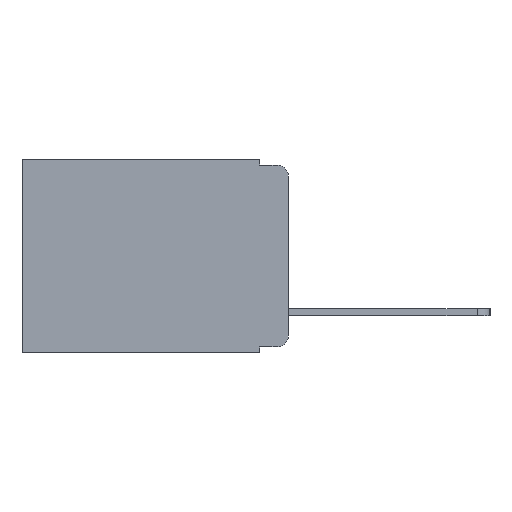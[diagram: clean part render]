
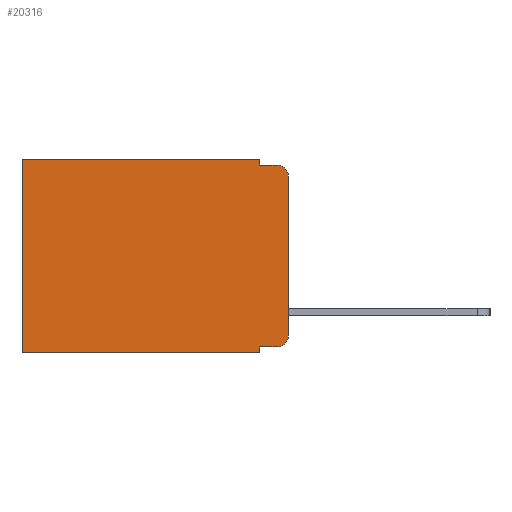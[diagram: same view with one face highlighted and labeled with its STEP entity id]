
A CAD part, left-side view. The second image highlights one B-rep face of the part: STEP entity #20316.
In plain terms, the highlighted planar face has unit normal (-1, 0, 0).
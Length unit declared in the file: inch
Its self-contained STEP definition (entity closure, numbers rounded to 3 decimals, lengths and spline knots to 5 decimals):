
#592 = ORIENTED_EDGE ( 'NONE', *, *, #4525, .F. ) ;
#769 = EDGE_CURVE ( 'NONE', #2695, #11790, #1768, .T. ) ;
#1333 = EDGE_CURVE ( 'NONE', #11790, #14523, #2235, .T. ) ;
#1568 = VECTOR ( 'NONE', #18440, 39.37008 ) ;
#1768 = LINE ( 'NONE', #15369, #18785 ) ;
#1835 = VECTOR ( 'NONE', #19156, 39.37008 ) ;
#2235 = LINE ( 'NONE', #2574, #6680 ) ;
#2326 = VERTEX_POINT ( 'NONE', #19909 ) ;
#2427 = VERTEX_POINT ( 'NONE', #18891 ) ;
#2574 = CARTESIAN_POINT ( 'NONE',  ( 0.298, 0., -0.343 ) ) ;
#2676 = DIRECTION ( 'NONE',  ( -1., 0., 0. ) ) ;
#2695 = VERTEX_POINT ( 'NONE', #8206 ) ;
#2753 = AXIS2_PLACEMENT_3D ( 'NONE', #18118, #8752, #19669 ) ;
#2941 = ORIENTED_EDGE ( 'NONE', *, *, #13127, .T. ) ;
#2972 = CIRCLE ( 'NONE', #10777, 0.02 ) ;
#3324 = DIRECTION ( 'NONE',  ( 1., 0., 0. ) ) ;
#3425 = ORIENTED_EDGE ( 'NONE', *, *, #16309, .T. ) ;
#3449 = CARTESIAN_POINT ( 'NONE',  ( 0.298, 0., 0. ) ) ;
#4099 = VECTOR ( 'NONE', #15192, 39.37008 ) ;
#4525 = EDGE_CURVE ( 'NONE', #5292, #13563, #7042, .T. ) ;
#4908 = DIRECTION ( 'NONE',  ( 0., 1., 0. ) ) ;
#5045 = ORIENTED_EDGE ( 'NONE', *, *, #5663, .F. ) ;
#5182 = PLANE ( 'NONE',  #19134 ) ;
#5292 = VERTEX_POINT ( 'NONE', #13034 ) ;
#5663 = EDGE_CURVE ( 'NONE', #17700, #12275, #8539, .T. ) ;
#6520 = VERTEX_POINT ( 'NONE', #13175 ) ;
#6633 = CARTESIAN_POINT ( 'NONE',  ( 0.298, 0.051, 0. ) ) ;
#6680 = VECTOR ( 'NONE', #4908, 39.37008 ) ;
#6870 = DIRECTION ( 'NONE',  ( 0., 0., -1. ) ) ;
#6920 = CARTESIAN_POINT ( 'NONE',  ( 0.298, 0., 0. ) ) ;
#7042 = LINE ( 'NONE', #10525, #1568 ) ;
#7335 = CARTESIAN_POINT ( 'NONE',  ( 0.298, 0.051, -0.333 ) ) ;
#7378 = CARTESIAN_POINT ( 'NONE',  ( 0.298, 0.051, -0.01 ) ) ;
#7644 = LINE ( 'NONE', #13726, #8873 ) ;
#7738 = LINE ( 'NONE', #7335, #19713 ) ;
#7903 = EDGE_CURVE ( 'NONE', #5292, #12275, #2972, .T. ) ;
#8206 = CARTESIAN_POINT ( 'NONE',  ( 0.298, 0.051, -0.333 ) ) ;
#8539 = LINE ( 'NONE', #7378, #4099 ) ;
#8565 = EDGE_CURVE ( 'NONE', #2326, #13563, #13370, .T. ) ;
#8752 = DIRECTION ( 'NONE',  ( -1., 0., 0. ) ) ;
#8873 = VECTOR ( 'NONE', #18473, 39.37008 ) ;
#9312 = FACE_OUTER_BOUND ( 'NONE', #13287, .T. ) ;
#9559 = CARTESIAN_POINT ( 'NONE',  ( 0.298, 0.473, -0.343 ) ) ;
#10337 = ORIENTED_EDGE ( 'NONE', *, *, #1333, .F. ) ;
#10525 = CARTESIAN_POINT ( 'NONE',  ( 0.298, 0., 0. ) ) ;
#10777 = AXIS2_PLACEMENT_3D ( 'NONE', #12347, #2676, #13936 ) ;
#10828 = ORIENTED_EDGE ( 'NONE', *, *, #8565, .T. ) ;
#10952 = CARTESIAN_POINT ( 'NONE',  ( 0.298, 0.051, -0.343 ) ) ;
#11535 = ORIENTED_EDGE ( 'NONE', *, *, #769, .F. ) ;
#11790 = VERTEX_POINT ( 'NONE', #10952 ) ;
#12275 = VERTEX_POINT ( 'NONE', #13337 ) ;
#12347 = CARTESIAN_POINT ( 'NONE',  ( 0.298, 0.02, -0.03 ) ) ;
#13034 = CARTESIAN_POINT ( 'NONE',  ( 0.298, 0., -0.03 ) ) ;
#13127 = EDGE_CURVE ( 'NONE', #2427, #14523, #7644, .T. ) ;
#13175 = CARTESIAN_POINT ( 'NONE',  ( 0.298, 0.051, 0. ) ) ;
#13287 = EDGE_LOOP ( 'NONE', ( #592, #15228, #5045, #15722, #13524, #2941, #10337, #11535, #3425, #10828 ) ) ;
#13337 = CARTESIAN_POINT ( 'NONE',  ( 0.298, 0.02, -0.01 ) ) ;
#13370 = CIRCLE ( 'NONE', #2753, 0.02 ) ;
#13524 = ORIENTED_EDGE ( 'NONE', *, *, #19018, .T. ) ;
#13563 = VERTEX_POINT ( 'NONE', #14945 ) ;
#13726 = CARTESIAN_POINT ( 'NONE',  ( 0.298, 0.473, 0. ) ) ;
#13936 = DIRECTION ( 'NONE',  ( 0., 0., -1. ) ) ;
#14523 = VERTEX_POINT ( 'NONE', #9559 ) ;
#14680 = LINE ( 'NONE', #6633, #1835 ) ;
#14754 = VECTOR ( 'NONE', #16418, 39.37008 ) ;
#14945 = CARTESIAN_POINT ( 'NONE',  ( 0.298, 0., -0.313 ) ) ;
#15192 = DIRECTION ( 'NONE',  ( 0., -1., 0. ) ) ;
#15228 = ORIENTED_EDGE ( 'NONE', *, *, #7903, .T. ) ;
#15241 = EDGE_CURVE ( 'NONE', #6520, #17700, #14680, .T. ) ;
#15369 = CARTESIAN_POINT ( 'NONE',  ( 0.298, 0.051, 0. ) ) ;
#15722 = ORIENTED_EDGE ( 'NONE', *, *, #15241, .F. ) ;
#16309 = EDGE_CURVE ( 'NONE', #2695, #2326, #7738, .T. ) ;
#16418 = DIRECTION ( 'NONE',  ( 0., 1., 0. ) ) ;
#16641 = DIRECTION ( 'NONE',  ( 0., 0., -1. ) ) ;
#17152 = CARTESIAN_POINT ( 'NONE',  ( 0.298, 0.051, -0.01 ) ) ;
#17700 = VERTEX_POINT ( 'NONE', #17152 ) ;
#18118 = CARTESIAN_POINT ( 'NONE',  ( 0.298, 0.02, -0.313 ) ) ;
#18323 = DIRECTION ( 'NONE',  ( 0., -1., 0. ) ) ;
#18440 = DIRECTION ( 'NONE',  ( 0., 0., -1. ) ) ;
#18473 = DIRECTION ( 'NONE',  ( 0., 0., -1. ) ) ;
#18785 = VECTOR ( 'NONE', #16641, 39.37008 ) ;
#18891 = CARTESIAN_POINT ( 'NONE',  ( 0.298, 0.473, 0. ) ) ;
#18916 = LINE ( 'NONE', #6920, #14754 ) ;
#19018 = EDGE_CURVE ( 'NONE', #6520, #2427, #18916, .T. ) ;
#19134 = AXIS2_PLACEMENT_3D ( 'NONE', #3449, #3324, #6870 ) ;
#19156 = DIRECTION ( 'NONE',  ( 0., 0., -1. ) ) ;
#19669 = DIRECTION ( 'NONE',  ( 0., 0., -1. ) ) ;
#19713 = VECTOR ( 'NONE', #18323, 39.37008 ) ;
#19909 = CARTESIAN_POINT ( 'NONE',  ( 0.298, 0.02, -0.333 ) ) ;
#20316 = ADVANCED_FACE ( 'NONE', ( #9312 ), #5182, .F. ) ;
